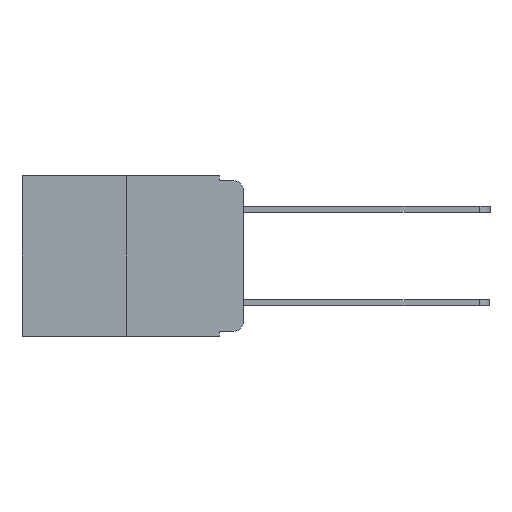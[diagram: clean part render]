
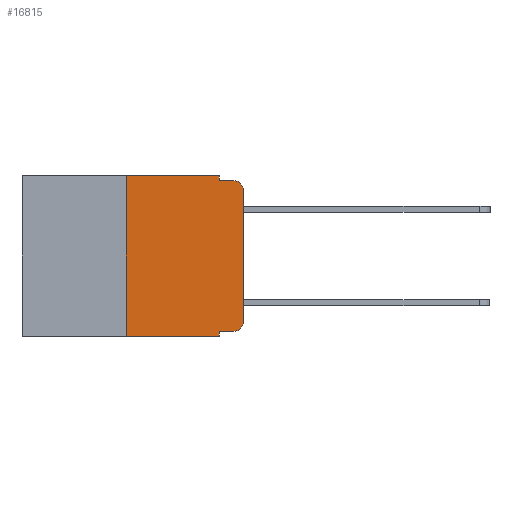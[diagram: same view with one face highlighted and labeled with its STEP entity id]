
A CAD part, left-side view. The second image highlights one B-rep face of the part: STEP entity #16815.
In plain terms, the highlighted planar face has unit normal (-1, 0, 0).
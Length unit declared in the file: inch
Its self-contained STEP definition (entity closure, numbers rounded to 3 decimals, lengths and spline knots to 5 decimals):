
#204 = CARTESIAN_POINT ( 'NONE',  ( 0., 0.02, -0.03 ) ) ;
#365 = EDGE_CURVE ( 'NONE', #6210, #12534, #7695, .T. ) ;
#709 = EDGE_CURVE ( 'NONE', #2512, #16818, #1242, .T. ) ;
#725 = VECTOR ( 'NONE', #14456, 39.37008 ) ;
#1112 = DIRECTION ( 'NONE',  ( -1., 0., 0. ) ) ;
#1242 = LINE ( 'NONE', #16831, #725 ) ;
#1282 = LINE ( 'NONE', #21738, #13787 ) ;
#1626 = CARTESIAN_POINT ( 'NONE',  ( 0., 0.051, -0.333 ) ) ;
#1757 = LINE ( 'NONE', #6386, #2272 ) ;
#1869 = DIRECTION ( 'NONE',  ( 0., 0., -1. ) ) ;
#2051 = VECTOR ( 'NONE', #21123, 39.37008 ) ;
#2272 = VECTOR ( 'NONE', #13205, 39.37008 ) ;
#2297 = ORIENTED_EDGE ( 'NONE', *, *, #11831, .F. ) ;
#2328 = CARTESIAN_POINT ( 'NONE',  ( 0., 0.25, 0. ) ) ;
#2448 = PLANE ( 'NONE',  #13518 ) ;
#2485 = EDGE_LOOP ( 'NONE', ( #13675, #11775, #2297, #13906, #14329, #11239, #20177, #6631, #8840, #8423 ) ) ;
#2488 = VECTOR ( 'NONE', #3074, 39.37008 ) ;
#2512 = VERTEX_POINT ( 'NONE', #1626 ) ;
#2555 = AXIS2_PLACEMENT_3D ( 'NONE', #15503, #1112, #19410 ) ;
#2832 = EDGE_CURVE ( 'NONE', #6598, #16877, #21926, .T. ) ;
#3074 = DIRECTION ( 'NONE',  ( 0., 0., 1. ) ) ;
#3336 = EDGE_CURVE ( 'NONE', #12534, #5830, #20129, .T. ) ;
#3400 = CARTESIAN_POINT ( 'NONE',  ( 0., 0.02, -0.01 ) ) ;
#4199 = DIRECTION ( 'NONE',  ( 1., 0., 0. ) ) ;
#4431 = CARTESIAN_POINT ( 'NONE',  ( 0., 0.051, -0.01 ) ) ;
#5227 = CIRCLE ( 'NONE', #8488, 0.02 ) ;
#5533 = CARTESIAN_POINT ( 'NONE',  ( 0., 0., 0. ) ) ;
#5733 = CARTESIAN_POINT ( 'NONE',  ( 0., 0.051, -0.01 ) ) ;
#5830 = VERTEX_POINT ( 'NONE', #18201 ) ;
#6210 = VERTEX_POINT ( 'NONE', #9021 ) ;
#6358 = CARTESIAN_POINT ( 'NONE',  ( 0., 0.25, 0. ) ) ;
#6386 = CARTESIAN_POINT ( 'NONE',  ( 0., 0.051, 0. ) ) ;
#6598 = VERTEX_POINT ( 'NONE', #6358 ) ;
#6620 = EDGE_CURVE ( 'NONE', #2512, #6210, #1282, .T. ) ;
#6631 = ORIENTED_EDGE ( 'NONE', *, *, #709, .F. ) ;
#7531 = DIRECTION ( 'NONE',  ( 0., -1., 0. ) ) ;
#7695 = CIRCLE ( 'NONE', #2555, 0.02 ) ;
#8370 = VECTOR ( 'NONE', #21944, 39.37008 ) ;
#8423 = ORIENTED_EDGE ( 'NONE', *, *, #365, .T. ) ;
#8488 = AXIS2_PLACEMENT_3D ( 'NONE', #204, #12098, #1869 ) ;
#8840 = ORIENTED_EDGE ( 'NONE', *, *, #6620, .T. ) ;
#9021 = CARTESIAN_POINT ( 'NONE',  ( 0., 0.02, -0.333 ) ) ;
#9364 = CARTESIAN_POINT ( 'NONE',  ( 0., 0.473, 0. ) ) ;
#11239 = ORIENTED_EDGE ( 'NONE', *, *, #16140, .F. ) ;
#11327 = LINE ( 'NONE', #19454, #11870 ) ;
#11775 = ORIENTED_EDGE ( 'NONE', *, *, #12597, .T. ) ;
#11831 = EDGE_CURVE ( 'NONE', #19031, #17872, #16170, .T. ) ;
#11870 = VECTOR ( 'NONE', #7531, 39.37008 ) ;
#11883 = CARTESIAN_POINT ( 'NONE',  ( 0., 0., -0.313 ) ) ;
#12098 = DIRECTION ( 'NONE',  ( -1., 0., 0. ) ) ;
#12126 = EDGE_CURVE ( 'NONE', #16877, #19031, #1757, .T. ) ;
#12534 = VERTEX_POINT ( 'NONE', #11883 ) ;
#12597 = EDGE_CURVE ( 'NONE', #5830, #17872, #5227, .T. ) ;
#12678 = CARTESIAN_POINT ( 'NONE',  ( 0., 0.051, -0.343 ) ) ;
#12725 = LINE ( 'NONE', #2328, #2051 ) ;
#13205 = DIRECTION ( 'NONE',  ( 0., 0., -1. ) ) ;
#13518 = AXIS2_PLACEMENT_3D ( 'NONE', #15938, #4199, #16103 ) ;
#13675 = ORIENTED_EDGE ( 'NONE', *, *, #3336, .T. ) ;
#13787 = VECTOR ( 'NONE', #16636, 39.37008 ) ;
#13906 = ORIENTED_EDGE ( 'NONE', *, *, #12126, .F. ) ;
#14329 = ORIENTED_EDGE ( 'NONE', *, *, #2832, .F. ) ;
#14456 = DIRECTION ( 'NONE',  ( 0., 0., -1. ) ) ;
#15503 = CARTESIAN_POINT ( 'NONE',  ( 0., 0.02, -0.313 ) ) ;
#15938 = CARTESIAN_POINT ( 'NONE',  ( 0., 0.473, 0. ) ) ;
#16103 = DIRECTION ( 'NONE',  ( 0., 0., -1. ) ) ;
#16140 = EDGE_CURVE ( 'NONE', #20280, #6598, #12725, .T. ) ;
#16170 = LINE ( 'NONE', #5733, #20729 ) ;
#16636 = DIRECTION ( 'NONE',  ( 0., -1., 0. ) ) ;
#16815 = ADVANCED_FACE ( 'NONE', ( #19933 ), #2448, .F. ) ;
#16818 = VERTEX_POINT ( 'NONE', #12678 ) ;
#16831 = CARTESIAN_POINT ( 'NONE',  ( 0., 0.051, 0. ) ) ;
#16877 = VERTEX_POINT ( 'NONE', #19705 ) ;
#17657 = DIRECTION ( 'NONE',  ( 0., -1., 0. ) ) ;
#17872 = VERTEX_POINT ( 'NONE', #3400 ) ;
#18201 = CARTESIAN_POINT ( 'NONE',  ( 0., 0., -0.03 ) ) ;
#18399 = CARTESIAN_POINT ( 'NONE',  ( 0., 0.25, -0.343 ) ) ;
#19031 = VERTEX_POINT ( 'NONE', #4431 ) ;
#19410 = DIRECTION ( 'NONE',  ( 0., 0., -1. ) ) ;
#19454 = CARTESIAN_POINT ( 'NONE',  ( 0., 0.473, -0.343 ) ) ;
#19705 = CARTESIAN_POINT ( 'NONE',  ( 0., 0.051, 0. ) ) ;
#19933 = FACE_OUTER_BOUND ( 'NONE', #2485, .T. ) ;
#20129 = LINE ( 'NONE', #5533, #2488 ) ;
#20177 = ORIENTED_EDGE ( 'NONE', *, *, #21971, .T. ) ;
#20280 = VERTEX_POINT ( 'NONE', #18399 ) ;
#20729 = VECTOR ( 'NONE', #17657, 39.37008 ) ;
#21123 = DIRECTION ( 'NONE',  ( 0., 0., 1. ) ) ;
#21738 = CARTESIAN_POINT ( 'NONE',  ( 0., 0.051, -0.333 ) ) ;
#21926 = LINE ( 'NONE', #9364, #8370 ) ;
#21944 = DIRECTION ( 'NONE',  ( 0., -1., 0. ) ) ;
#21971 = EDGE_CURVE ( 'NONE', #20280, #16818, #11327, .T. ) ;
